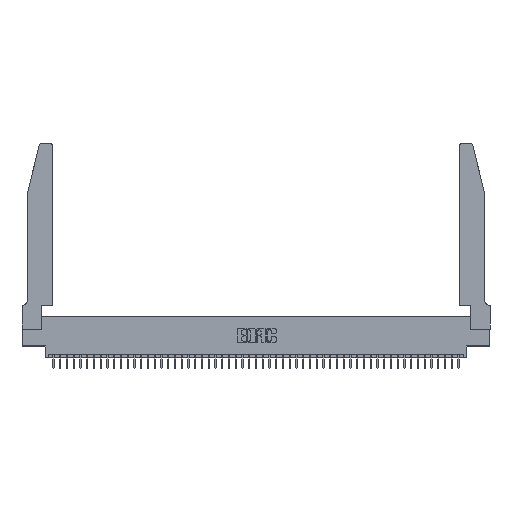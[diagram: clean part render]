
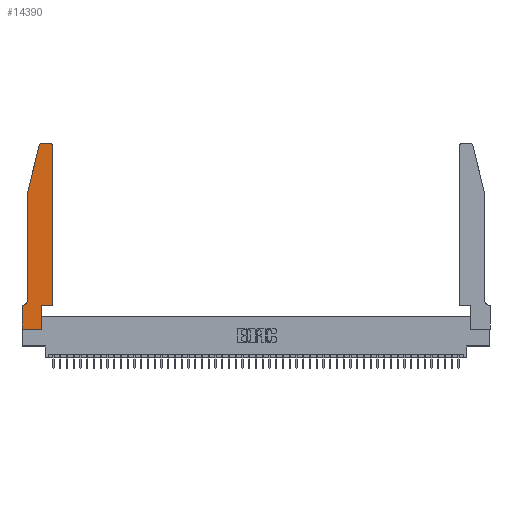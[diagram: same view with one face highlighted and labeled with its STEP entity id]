
A CAD part, top view. The second image highlights one B-rep face of the part: STEP entity #14390.
In plain terms, the highlighted planar face has unit normal (0, 0, 1).
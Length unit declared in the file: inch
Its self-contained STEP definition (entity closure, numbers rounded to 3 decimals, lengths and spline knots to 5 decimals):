
#854 = VECTOR ( 'NONE', #12997, 39.37008 ) ;
#1308 = CARTESIAN_POINT ( 'NONE',  ( 0.4205, 2.75, 0.37 ) ) ;
#1578 = VECTOR ( 'NONE', #40336, 39.37008 ) ;
#1669 = VERTEX_POINT ( 'NONE', #6629 ) ;
#1927 = LINE ( 'NONE', #7094, #39564 ) ;
#2157 = DIRECTION ( 'NONE',  ( 0., 0., -1. ) ) ;
#2518 = EDGE_CURVE ( 'NONE', #10784, #20688, #6764, .T. ) ;
#3893 = LINE ( 'NONE', #13335, #854 ) ;
#5105 = ORIENTED_EDGE ( 'NONE', *, *, #16876, .T. ) ;
#5364 = CARTESIAN_POINT ( 'NONE',  ( 0.4505, 0.35, 0.37 ) ) ;
#5686 = VECTOR ( 'NONE', #15366, 39.37008 ) ;
#5812 = AXIS2_PLACEMENT_3D ( 'NONE', #22586, #45497, #34284 ) ;
#6629 = CARTESIAN_POINT ( 'NONE',  ( 0.0055, 0.35, 0.37 ) ) ;
#6764 = CIRCLE ( 'NONE', #31582, 0.03 ) ;
#6831 = CARTESIAN_POINT ( 'NONE',  ( 0.4505, 2.72, 0.37 ) ) ;
#7094 = CARTESIAN_POINT ( 'NONE',  ( 0.2605, 2.75, 0.37 ) ) ;
#7328 = CIRCLE ( 'NONE', #22658, 0.03 ) ;
#7546 = CARTESIAN_POINT ( 'NONE',  ( 0.2865, 0.35, 0.37 ) ) ;
#8629 = ORIENTED_EDGE ( 'NONE', *, *, #28513, .T. ) ;
#9170 = DIRECTION ( 'NONE',  ( 1., 0., 0. ) ) ;
#9716 = VECTOR ( 'NONE', #33460, 39.37008 ) ;
#9728 = ORIENTED_EDGE ( 'NONE', *, *, #2518, .T. ) ;
#9808 = VERTEX_POINT ( 'NONE', #38772 ) ;
#10706 = CARTESIAN_POINT ( 'NONE',  ( 0.4505, 0.35, 0.37 ) ) ;
#10784 = VERTEX_POINT ( 'NONE', #6831 ) ;
#11779 = CARTESIAN_POINT ( 'NONE',  ( 0.2865, 0., 0.37 ) ) ;
#12117 = ORIENTED_EDGE ( 'NONE', *, *, #12385, .T. ) ;
#12385 = EDGE_CURVE ( 'NONE', #44200, #47931, #3893, .T. ) ;
#12919 = EDGE_CURVE ( 'NONE', #20306, #44200, #44793, .T. ) ;
#12997 = DIRECTION ( 'NONE',  ( 1., 0., 0. ) ) ;
#13335 = CARTESIAN_POINT ( 'NONE',  ( 0., 0., 0.37 ) ) ;
#13733 = EDGE_LOOP ( 'NONE', ( #23910, #39706, #40882, #22268, #5105, #30055, #46822, #12117, #8629, #32291, #38736, #9728 ) ) ;
#14390 = ADVANCED_FACE ( 'NONE', ( #34313 ), #14415, .T. ) ;
#14415 = PLANE ( 'NONE',  #5812 ) ;
#15366 = DIRECTION ( 'NONE',  ( 0., 1., 0. ) ) ;
#16013 = VERTEX_POINT ( 'NONE', #47883 ) ;
#16267 = CARTESIAN_POINT ( 'NONE',  ( 0.0755, 2., 0.37 ) ) ;
#16308 = CARTESIAN_POINT ( 'NONE',  ( 0.284, 2.72, 0.37 ) ) ;
#16451 = EDGE_CURVE ( 'NONE', #20688, #9808, #1927, .T. ) ;
#16876 = EDGE_CURVE ( 'NONE', #40468, #1669, #45614, .T. ) ;
#17422 = DIRECTION ( 'NONE',  ( -1., 0., 0. ) ) ;
#17657 = CARTESIAN_POINT ( 'NONE',  ( 0.0755, 2., 0.37 ) ) ;
#17964 = EDGE_CURVE ( 'NONE', #37742, #40468, #31614, .T. ) ;
#20006 = CARTESIAN_POINT ( 'NONE',  ( 0., 0., 0.37 ) ) ;
#20306 = VERTEX_POINT ( 'NONE', #42419 ) ;
#20473 = DIRECTION ( 'NONE',  ( 1., 0., 0. ) ) ;
#20688 = VERTEX_POINT ( 'NONE', #1308 ) ;
#20703 = EDGE_CURVE ( 'NONE', #45036, #10784, #21011, .T. ) ;
#21011 = LINE ( 'NONE', #5364, #1578 ) ;
#21561 = DIRECTION ( 'NONE',  ( -1., 0., 0. ) ) ;
#22227 = EDGE_CURVE ( 'NONE', #16013, #45036, #40345, .T. ) ;
#22268 = ORIENTED_EDGE ( 'NONE', *, *, #17964, .T. ) ;
#22586 = CARTESIAN_POINT ( 'NONE',  ( 0., 0.35, 0.37 ) ) ;
#22658 = AXIS2_PLACEMENT_3D ( 'NONE', #16308, #28573, #9170 ) ;
#22769 = VECTOR ( 'NONE', #37944, 39.37008 ) ;
#23910 = ORIENTED_EDGE ( 'NONE', *, *, #16451, .T. ) ;
#23949 = LINE ( 'NONE', #7546, #5686 ) ;
#26400 = VERTEX_POINT ( 'NONE', #32510 ) ;
#27220 = VECTOR ( 'NONE', #43797, 39.37008 ) ;
#28232 = CARTESIAN_POINT ( 'NONE',  ( 0.0755, 0.42, 0.37 ) ) ;
#28267 = EDGE_CURVE ( 'NONE', #26400, #37742, #31871, .T. ) ;
#28513 = EDGE_CURVE ( 'NONE', #47931, #16013, #23949, .T. ) ;
#28573 = DIRECTION ( 'NONE',  ( 0., 0., 1. ) ) ;
#28954 = LINE ( 'NONE', #40555, #45909 ) ;
#30055 = ORIENTED_EDGE ( 'NONE', *, *, #33315, .T. ) ;
#31582 = AXIS2_PLACEMENT_3D ( 'NONE', #47459, #32392, #20473 ) ;
#31614 = LINE ( 'NONE', #17657, #9716 ) ;
#31871 = LINE ( 'NONE', #45277, #22769 ) ;
#32291 = ORIENTED_EDGE ( 'NONE', *, *, #22227, .T. ) ;
#32392 = DIRECTION ( 'NONE',  ( 0., 0., 1. ) ) ;
#32510 = CARTESIAN_POINT ( 'NONE',  ( 0.25487, 2.72718, 0.37 ) ) ;
#32902 = CARTESIAN_POINT ( 'NONE',  ( 0.0055, 0.42, 0.37 ) ) ;
#33315 = EDGE_CURVE ( 'NONE', #1669, #20306, #28954, .T. ) ;
#33460 = DIRECTION ( 'NONE',  ( 0., -1., 0. ) ) ;
#34284 = DIRECTION ( 'NONE',  ( 1., 0., 0. ) ) ;
#34313 = FACE_OUTER_BOUND ( 'NONE', #13733, .T. ) ;
#37318 = VECTOR ( 'NONE', #41621, 39.37008 ) ;
#37742 = VERTEX_POINT ( 'NONE', #16267 ) ;
#37944 = DIRECTION ( 'NONE',  ( -0.239, -0.971, 0. ) ) ;
#38736 = ORIENTED_EDGE ( 'NONE', *, *, #20703, .T. ) ;
#38772 = CARTESIAN_POINT ( 'NONE',  ( 0.284, 2.75, 0.37 ) ) ;
#39564 = VECTOR ( 'NONE', #42257, 39.37008 ) ;
#39706 = ORIENTED_EDGE ( 'NONE', *, *, #44895, .T. ) ;
#40336 = DIRECTION ( 'NONE',  ( 0., 1., 0. ) ) ;
#40345 = LINE ( 'NONE', #10706, #37318 ) ;
#40468 = VERTEX_POINT ( 'NONE', #28232 ) ;
#40555 = CARTESIAN_POINT ( 'NONE',  ( 0.0755, 0.35, 0.37 ) ) ;
#40882 = ORIENTED_EDGE ( 'NONE', *, *, #28267, .T. ) ;
#41621 = DIRECTION ( 'NONE',  ( 1., 0., 0. ) ) ;
#42257 = DIRECTION ( 'NONE',  ( -1., 0., 0. ) ) ;
#42419 = CARTESIAN_POINT ( 'NONE',  ( 0., 0.35, 0.37 ) ) ;
#43797 = DIRECTION ( 'NONE',  ( 0., -1., 0. ) ) ;
#44200 = VERTEX_POINT ( 'NONE', #47434 ) ;
#44656 = CARTESIAN_POINT ( 'NONE',  ( 0.4505, 0.35, 0.37 ) ) ;
#44793 = LINE ( 'NONE', #20006, #27220 ) ;
#44895 = EDGE_CURVE ( 'NONE', #9808, #26400, #7328, .T. ) ;
#45036 = VERTEX_POINT ( 'NONE', #44656 ) ;
#45277 = CARTESIAN_POINT ( 'NONE',  ( 0.0755, 2., 0.37 ) ) ;
#45497 = DIRECTION ( 'NONE',  ( 0., 0., 1. ) ) ;
#45614 = CIRCLE ( 'NONE', #48209, 0.07 ) ;
#45909 = VECTOR ( 'NONE', #21561, 39.37008 ) ;
#46822 = ORIENTED_EDGE ( 'NONE', *, *, #12919, .T. ) ;
#47434 = CARTESIAN_POINT ( 'NONE',  ( 0., 0., 0.37 ) ) ;
#47459 = CARTESIAN_POINT ( 'NONE',  ( 0.4205, 2.72, 0.37 ) ) ;
#47883 = CARTESIAN_POINT ( 'NONE',  ( 0.2865, 0.35, 0.37 ) ) ;
#47931 = VERTEX_POINT ( 'NONE', #11779 ) ;
#48209 = AXIS2_PLACEMENT_3D ( 'NONE', #32902, #2157, #17422 ) ;
